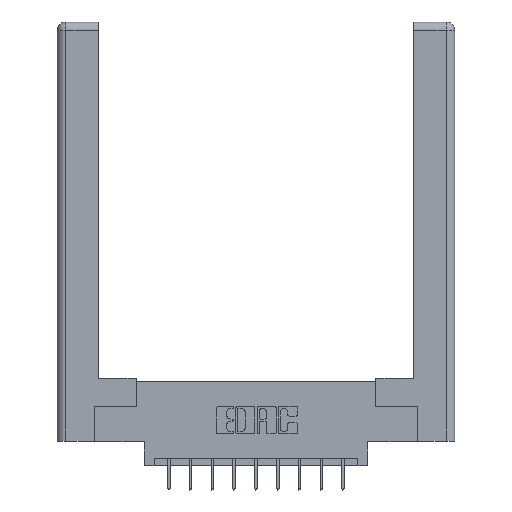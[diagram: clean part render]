
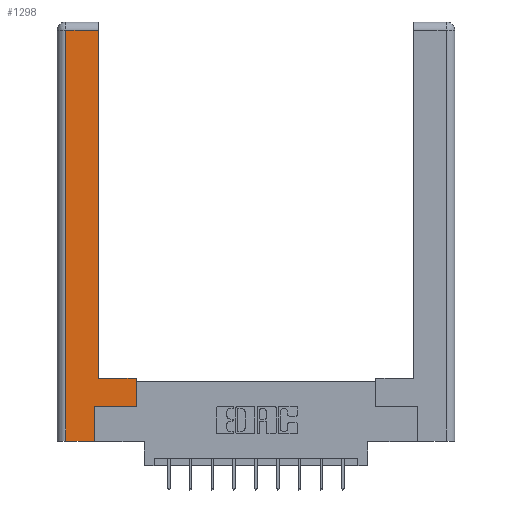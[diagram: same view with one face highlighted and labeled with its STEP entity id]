
A CAD part, top view. The second image highlights one B-rep face of the part: STEP entity #1298.
In plain terms, the highlighted planar face has unit normal (0, 0, 1).
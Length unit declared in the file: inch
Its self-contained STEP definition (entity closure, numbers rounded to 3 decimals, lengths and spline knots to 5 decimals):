
#70 = DIRECTION ( 'NONE',  ( 0., 0., -1. ) ) ;
#163 = ORIENTED_EDGE ( 'NONE', *, *, #3070, .T. ) ;
#183 = CARTESIAN_POINT ( 'NONE',  ( 0.265, 0.245, 0. ) ) ;
#440 = ORIENTED_EDGE ( 'NONE', *, *, #8582, .T. ) ;
#772 = DIRECTION ( 'NONE',  ( 0., -1., 0. ) ) ;
#1162 = DIRECTION ( 'NONE',  ( 0., 1., 0. ) ) ;
#1298 = ADVANCED_FACE ( 'NONE', ( #2982 ), #3510, .F. ) ;
#1439 = EDGE_CURVE ( 'NONE', #13306, #10833, #8685, .T. ) ;
#1457 = VECTOR ( 'NONE', #8522, 39.37008 ) ;
#1525 = VECTOR ( 'NONE', #12332, 39.37008 ) ;
#1599 = CARTESIAN_POINT ( 'NONE',  ( 0.565, 0.45, 0. ) ) ;
#1805 = DIRECTION ( 'NONE',  ( -1., 0., 0. ) ) ;
#1947 = LINE ( 'NONE', #12599, #3293 ) ;
#1995 = VECTOR ( 'NONE', #4747, 39.37008 ) ;
#2037 = LINE ( 'NONE', #3978, #13272 ) ;
#2601 = CARTESIAN_POINT ( 'NONE',  ( 0.0615, 2.94, 0. ) ) ;
#2966 = VERTEX_POINT ( 'NONE', #12400 ) ;
#2982 = FACE_OUTER_BOUND ( 'NONE', #6093, .T. ) ;
#3070 = EDGE_CURVE ( 'NONE', #11327, #8154, #12167, .T. ) ;
#3293 = VECTOR ( 'NONE', #772, 39.37008 ) ;
#3510 = PLANE ( 'NONE',  #10604 ) ;
#3978 = CARTESIAN_POINT ( 'NONE',  ( 0.265, 0., 0. ) ) ;
#4171 = CARTESIAN_POINT ( 'NONE',  ( 0.565, 0.245, 0. ) ) ;
#4400 = CARTESIAN_POINT ( 'NONE',  ( 0.295, 0.45, 0. ) ) ;
#4747 = DIRECTION ( 'NONE',  ( -1., 0., 0. ) ) ;
#5022 = DIRECTION ( 'NONE',  ( 1., 0., 0. ) ) ;
#5209 = ORIENTED_EDGE ( 'NONE', *, *, #11153, .T. ) ;
#5259 = VECTOR ( 'NONE', #1162, 39.37008 ) ;
#5336 = EDGE_CURVE ( 'NONE', #2966, #6733, #12750, .T. ) ;
#5403 = CARTESIAN_POINT ( 'NONE',  ( 0.265, 0.245, 0. ) ) ;
#5794 = LINE ( 'NONE', #1599, #1525 ) ;
#5961 = CARTESIAN_POINT ( 'NONE',  ( 0.295, 3., 0. ) ) ;
#6093 = EDGE_LOOP ( 'NONE', ( #13494, #13449, #440, #10845, #6316, #11681, #5209, #163 ) ) ;
#6287 = CARTESIAN_POINT ( 'NONE',  ( 0.295, 0.45, 0. ) ) ;
#6316 = ORIENTED_EDGE ( 'NONE', *, *, #5336, .T. ) ;
#6621 = VERTEX_POINT ( 'NONE', #9946 ) ;
#6733 = VERTEX_POINT ( 'NONE', #183 ) ;
#6975 = VECTOR ( 'NONE', #10379, 39.37008 ) ;
#7702 = DIRECTION ( 'NONE',  ( -1., 0., 0. ) ) ;
#8023 = EDGE_CURVE ( 'NONE', #6733, #6621, #8786, .T. ) ;
#8099 = CARTESIAN_POINT ( 'NONE',  ( 0.295, 2.94, 0. ) ) ;
#8154 = VERTEX_POINT ( 'NONE', #4400 ) ;
#8225 = CARTESIAN_POINT ( 'NONE',  ( 0.565, 0.45, 0. ) ) ;
#8522 = DIRECTION ( 'NONE',  ( 1., 0., 0. ) ) ;
#8582 = EDGE_CURVE ( 'NONE', #10833, #10934, #1947, .T. ) ;
#8685 = LINE ( 'NONE', #2601, #1995 ) ;
#8786 = LINE ( 'NONE', #4171, #1457 ) ;
#9070 = VECTOR ( 'NONE', #1805, 39.37008 ) ;
#9667 = CARTESIAN_POINT ( 'NONE',  ( 0.0615, 0., 0. ) ) ;
#9946 = CARTESIAN_POINT ( 'NONE',  ( 0.565, 0.245, 0. ) ) ;
#10379 = DIRECTION ( 'NONE',  ( 0., 1., 0. ) ) ;
#10604 = AXIS2_PLACEMENT_3D ( 'NONE', #11131, #70, #7702 ) ;
#10833 = VERTEX_POINT ( 'NONE', #13791 ) ;
#10845 = ORIENTED_EDGE ( 'NONE', *, *, #11243, .T. ) ;
#10934 = VERTEX_POINT ( 'NONE', #9667 ) ;
#11131 = CARTESIAN_POINT ( 'NONE',  ( 0., 0., 0. ) ) ;
#11153 = EDGE_CURVE ( 'NONE', #6621, #11327, #5794, .T. ) ;
#11243 = EDGE_CURVE ( 'NONE', #10934, #2966, #2037, .T. ) ;
#11327 = VERTEX_POINT ( 'NONE', #8225 ) ;
#11681 = ORIENTED_EDGE ( 'NONE', *, *, #8023, .T. ) ;
#12167 = LINE ( 'NONE', #6287, #9070 ) ;
#12234 = LINE ( 'NONE', #5961, #6975 ) ;
#12320 = EDGE_CURVE ( 'NONE', #8154, #13306, #12234, .T. ) ;
#12332 = DIRECTION ( 'NONE',  ( 0., 1., 0. ) ) ;
#12400 = CARTESIAN_POINT ( 'NONE',  ( 0.265, 0., 0. ) ) ;
#12599 = CARTESIAN_POINT ( 'NONE',  ( 0.0615, 0., 0. ) ) ;
#12750 = LINE ( 'NONE', #5403, #5259 ) ;
#13272 = VECTOR ( 'NONE', #5022, 39.37008 ) ;
#13306 = VERTEX_POINT ( 'NONE', #8099 ) ;
#13449 = ORIENTED_EDGE ( 'NONE', *, *, #1439, .T. ) ;
#13494 = ORIENTED_EDGE ( 'NONE', *, *, #12320, .T. ) ;
#13791 = CARTESIAN_POINT ( 'NONE',  ( 0.0615, 2.94, 0. ) ) ;
